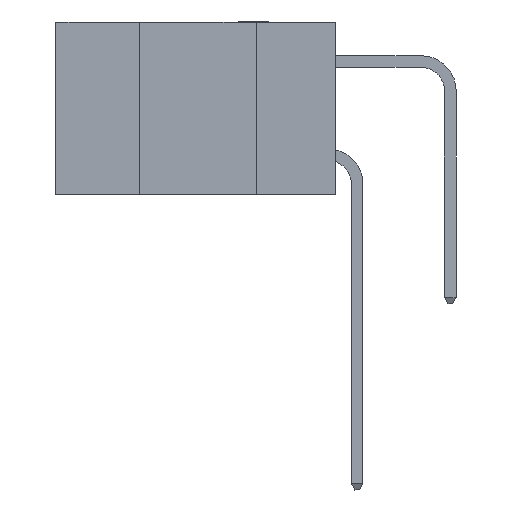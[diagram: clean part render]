
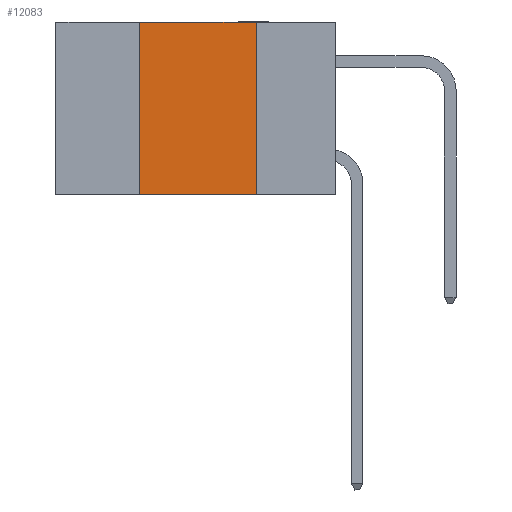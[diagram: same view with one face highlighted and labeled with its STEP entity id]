
A CAD part, left-side view. The second image highlights one B-rep face of the part: STEP entity #12083.
In plain terms, the highlighted planar face has unit normal (-1, 0, 0).
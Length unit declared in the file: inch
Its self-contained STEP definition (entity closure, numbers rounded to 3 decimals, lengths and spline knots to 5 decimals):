
#1370 = VECTOR ( 'NONE', #20349, 39.37008 ) ;
#1702 = ORIENTED_EDGE ( 'NONE', *, *, #8549, .F. ) ;
#1724 = CARTESIAN_POINT ( 'NONE',  ( 0., 0.6, 0. ) ) ;
#2493 = VECTOR ( 'NONE', #13101, 39.37008 ) ;
#3986 = VECTOR ( 'NONE', #19754, 39.37008 ) ;
#4292 = DIRECTION ( 'NONE',  ( 0., 0., 1. ) ) ;
#5613 = CARTESIAN_POINT ( 'NONE',  ( 0., 0.17, 0. ) ) ;
#5629 = EDGE_CURVE ( 'NONE', #15205, #7329, #15710, .T. ) ;
#6981 = FACE_OUTER_BOUND ( 'NONE', #11480, .T. ) ;
#7242 = CARTESIAN_POINT ( 'NONE',  ( 0., 0.6, -0.37 ) ) ;
#7329 = VERTEX_POINT ( 'NONE', #17952 ) ;
#7341 = LINE ( 'NONE', #1724, #2493 ) ;
#7565 = CARTESIAN_POINT ( 'NONE',  ( 0., 0.42, 0. ) ) ;
#8549 = EDGE_CURVE ( 'NONE', #21114, #13720, #12727, .T. ) ;
#8555 = AXIS2_PLACEMENT_3D ( 'NONE', #8813, #20202, #10535 ) ;
#8813 = CARTESIAN_POINT ( 'NONE',  ( 0., 0.6, 0. ) ) ;
#8827 = EDGE_CURVE ( 'NONE', #13720, #15205, #7341, .T. ) ;
#10535 = DIRECTION ( 'NONE',  ( 0., 0., -1. ) ) ;
#11480 = EDGE_LOOP ( 'NONE', ( #19775, #19922, #1702, #16821 ) ) ;
#11842 = CARTESIAN_POINT ( 'NONE',  ( 0., 0.42, -0.37 ) ) ;
#12054 = EDGE_CURVE ( 'NONE', #21114, #7329, #13848, .T. ) ;
#12083 = ADVANCED_FACE ( 'NONE', ( #6981 ), #13724, .F. ) ;
#12727 = LINE ( 'NONE', #7565, #15773 ) ;
#13101 = DIRECTION ( 'NONE',  ( 0., -1., 0. ) ) ;
#13276 = CARTESIAN_POINT ( 'NONE',  ( 0., 0.42, 0. ) ) ;
#13720 = VERTEX_POINT ( 'NONE', #13276 ) ;
#13724 = PLANE ( 'NONE',  #8555 ) ;
#13848 = LINE ( 'NONE', #7242, #1370 ) ;
#15205 = VERTEX_POINT ( 'NONE', #5613 ) ;
#15710 = LINE ( 'NONE', #16624, #3986 ) ;
#15773 = VECTOR ( 'NONE', #4292, 39.37008 ) ;
#16624 = CARTESIAN_POINT ( 'NONE',  ( 0., 0.17, 0. ) ) ;
#16821 = ORIENTED_EDGE ( 'NONE', *, *, #12054, .T. ) ;
#17952 = CARTESIAN_POINT ( 'NONE',  ( 0., 0.17, -0.37 ) ) ;
#19754 = DIRECTION ( 'NONE',  ( 0., 0., -1. ) ) ;
#19775 = ORIENTED_EDGE ( 'NONE', *, *, #5629, .F. ) ;
#19922 = ORIENTED_EDGE ( 'NONE', *, *, #8827, .F. ) ;
#20202 = DIRECTION ( 'NONE',  ( 1., 0., 0. ) ) ;
#20349 = DIRECTION ( 'NONE',  ( 0., -1., 0. ) ) ;
#21114 = VERTEX_POINT ( 'NONE', #11842 ) ;
